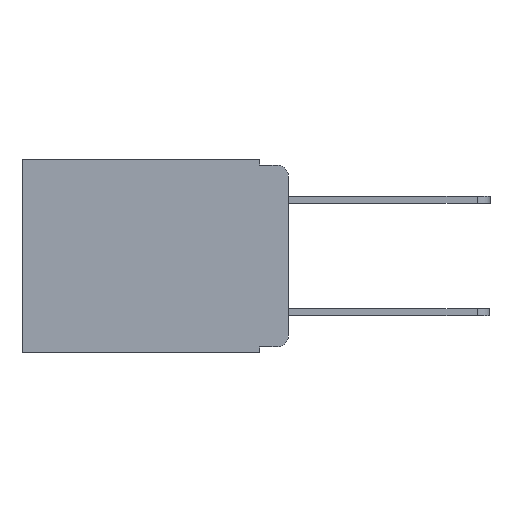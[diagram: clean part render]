
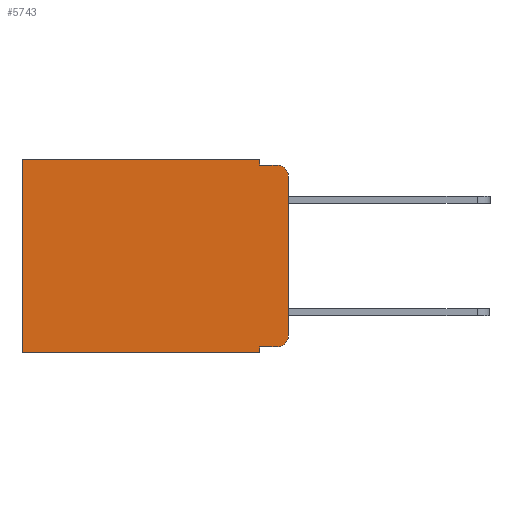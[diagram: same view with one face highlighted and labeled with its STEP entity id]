
A CAD part, left-side view. The second image highlights one B-rep face of the part: STEP entity #5743.
In plain terms, the highlighted planar face has unit normal (-1, 0, 0).
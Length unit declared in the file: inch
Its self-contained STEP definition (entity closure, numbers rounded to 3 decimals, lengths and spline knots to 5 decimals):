
#79 = CARTESIAN_POINT ( 'NONE',  ( 0.298, 0.051, -0.333 ) ) ;
#660 = DIRECTION ( 'NONE',  ( 0., 0., -1. ) ) ;
#1159 = ORIENTED_EDGE ( 'NONE', *, *, #6145, .T. ) ;
#2103 = DIRECTION ( 'NONE',  ( 0., 1., 0. ) ) ;
#2318 = EDGE_CURVE ( 'NONE', #18016, #14192, #8367, .T. ) ;
#2459 = VECTOR ( 'NONE', #17806, 39.37008 ) ;
#2980 = VECTOR ( 'NONE', #17738, 39.37008 ) ;
#3511 = VECTOR ( 'NONE', #16676, 39.37008 ) ;
#4160 = VECTOR ( 'NONE', #9508, 39.37008 ) ;
#4167 = DIRECTION ( 'NONE',  ( 1., 0., 0. ) ) ;
#4382 = DIRECTION ( 'NONE',  ( -1., 0., 0. ) ) ;
#4666 = CARTESIAN_POINT ( 'NONE',  ( 0.298, 0., 0. ) ) ;
#4980 = VECTOR ( 'NONE', #5130, 39.37008 ) ;
#5038 = CARTESIAN_POINT ( 'NONE',  ( 0.298, 0., 0. ) ) ;
#5130 = DIRECTION ( 'NONE',  ( 0., 0., -1. ) ) ;
#5136 = EDGE_CURVE ( 'NONE', #8170, #14712, #16563, .T. ) ;
#5175 = ORIENTED_EDGE ( 'NONE', *, *, #8065, .T. ) ;
#5508 = CARTESIAN_POINT ( 'NONE',  ( 0.298, 0.051, 0. ) ) ;
#5583 = FACE_OUTER_BOUND ( 'NONE', #22237, .T. ) ;
#5743 = ADVANCED_FACE ( 'NONE', ( #5583 ), #17882, .F. ) ;
#6039 = EDGE_CURVE ( 'NONE', #17447, #8866, #18139, .T. ) ;
#6145 = EDGE_CURVE ( 'NONE', #14192, #11083, #6713, .T. ) ;
#6178 = CARTESIAN_POINT ( 'NONE',  ( 0.298, 0.02, -0.333 ) ) ;
#6273 = EDGE_CURVE ( 'NONE', #8066, #11083, #9246, .T. ) ;
#6628 = CIRCLE ( 'NONE', #10833, 0.02 ) ;
#6713 = CIRCLE ( 'NONE', #12225, 0.02 ) ;
#7819 = VECTOR ( 'NONE', #2103, 39.37008 ) ;
#8065 = EDGE_CURVE ( 'NONE', #8066, #14712, #6628, .T. ) ;
#8066 = VERTEX_POINT ( 'NONE', #21713 ) ;
#8075 = ORIENTED_EDGE ( 'NONE', *, *, #6039, .T. ) ;
#8170 = VERTEX_POINT ( 'NONE', #16962 ) ;
#8367 = LINE ( 'NONE', #12166, #3511 ) ;
#8383 = CARTESIAN_POINT ( 'NONE',  ( 0.298, 0.051, -0.01 ) ) ;
#8634 = ORIENTED_EDGE ( 'NONE', *, *, #16282, .F. ) ;
#8711 = VERTEX_POINT ( 'NONE', #13258 ) ;
#8866 = VERTEX_POINT ( 'NONE', #17090 ) ;
#9246 = LINE ( 'NONE', #5038, #4980 ) ;
#9363 = CARTESIAN_POINT ( 'NONE',  ( 0.298, 0., 0. ) ) ;
#9378 = DIRECTION ( 'NONE',  ( 0., 1., 0. ) ) ;
#9430 = ORIENTED_EDGE ( 'NONE', *, *, #6273, .F. ) ;
#9508 = DIRECTION ( 'NONE',  ( 0., 0., -1. ) ) ;
#10155 = LINE ( 'NONE', #21412, #19851 ) ;
#10255 = ORIENTED_EDGE ( 'NONE', *, *, #2318, .T. ) ;
#10544 = CARTESIAN_POINT ( 'NONE',  ( 0.298, 0.473, 0. ) ) ;
#10833 = AXIS2_PLACEMENT_3D ( 'NONE', #14953, #4382, #16665 ) ;
#11083 = VERTEX_POINT ( 'NONE', #12920 ) ;
#11505 = CARTESIAN_POINT ( 'NONE',  ( 0.298, 0.051, 0. ) ) ;
#12166 = CARTESIAN_POINT ( 'NONE',  ( 0.298, 0.051, -0.333 ) ) ;
#12225 = AXIS2_PLACEMENT_3D ( 'NONE', #20763, #20986, #20932 ) ;
#12430 = LINE ( 'NONE', #9363, #7819 ) ;
#12436 = LINE ( 'NONE', #11505, #17014 ) ;
#12692 = EDGE_CURVE ( 'NONE', #17564, #8170, #21091, .T. ) ;
#12920 = CARTESIAN_POINT ( 'NONE',  ( 0.298, 0., -0.313 ) ) ;
#13258 = CARTESIAN_POINT ( 'NONE',  ( 0.298, 0.051, -0.343 ) ) ;
#13571 = EDGE_CURVE ( 'NONE', #18016, #8711, #12436, .T. ) ;
#14192 = VERTEX_POINT ( 'NONE', #6178 ) ;
#14712 = VERTEX_POINT ( 'NONE', #19790 ) ;
#14953 = CARTESIAN_POINT ( 'NONE',  ( 0.298, 0.02, -0.03 ) ) ;
#15104 = ORIENTED_EDGE ( 'NONE', *, *, #5136, .F. ) ;
#16282 = EDGE_CURVE ( 'NONE', #8711, #8866, #10155, .T. ) ;
#16563 = LINE ( 'NONE', #8383, #2459 ) ;
#16665 = DIRECTION ( 'NONE',  ( 0., 0., -1. ) ) ;
#16676 = DIRECTION ( 'NONE',  ( 0., -1., 0. ) ) ;
#16704 = ORIENTED_EDGE ( 'NONE', *, *, #20766, .T. ) ;
#16962 = CARTESIAN_POINT ( 'NONE',  ( 0.298, 0.051, -0.01 ) ) ;
#17014 = VECTOR ( 'NONE', #660, 39.37008 ) ;
#17090 = CARTESIAN_POINT ( 'NONE',  ( 0.298, 0.473, -0.343 ) ) ;
#17264 = AXIS2_PLACEMENT_3D ( 'NONE', #4666, #4167, #21888 ) ;
#17447 = VERTEX_POINT ( 'NONE', #18049 ) ;
#17564 = VERTEX_POINT ( 'NONE', #21813 ) ;
#17738 = DIRECTION ( 'NONE',  ( 0., 0., -1. ) ) ;
#17806 = DIRECTION ( 'NONE',  ( 0., -1., 0. ) ) ;
#17882 = PLANE ( 'NONE',  #17264 ) ;
#18016 = VERTEX_POINT ( 'NONE', #79 ) ;
#18049 = CARTESIAN_POINT ( 'NONE',  ( 0.298, 0.473, 0. ) ) ;
#18139 = LINE ( 'NONE', #10544, #4160 ) ;
#18322 = ORIENTED_EDGE ( 'NONE', *, *, #13571, .F. ) ;
#19790 = CARTESIAN_POINT ( 'NONE',  ( 0.298, 0.02, -0.01 ) ) ;
#19851 = VECTOR ( 'NONE', #9378, 39.37008 ) ;
#20205 = ORIENTED_EDGE ( 'NONE', *, *, #12692, .F. ) ;
#20763 = CARTESIAN_POINT ( 'NONE',  ( 0.298, 0.02, -0.313 ) ) ;
#20766 = EDGE_CURVE ( 'NONE', #17564, #17447, #12430, .T. ) ;
#20932 = DIRECTION ( 'NONE',  ( 0., 0., -1. ) ) ;
#20986 = DIRECTION ( 'NONE',  ( -1., 0., 0. ) ) ;
#21091 = LINE ( 'NONE', #5508, #2980 ) ;
#21412 = CARTESIAN_POINT ( 'NONE',  ( 0.298, 0., -0.343 ) ) ;
#21713 = CARTESIAN_POINT ( 'NONE',  ( 0.298, 0., -0.03 ) ) ;
#21813 = CARTESIAN_POINT ( 'NONE',  ( 0.298, 0.051, 0. ) ) ;
#21888 = DIRECTION ( 'NONE',  ( 0., 0., -1. ) ) ;
#22237 = EDGE_LOOP ( 'NONE', ( #9430, #5175, #15104, #20205, #16704, #8075, #8634, #18322, #10255, #1159 ) ) ;
